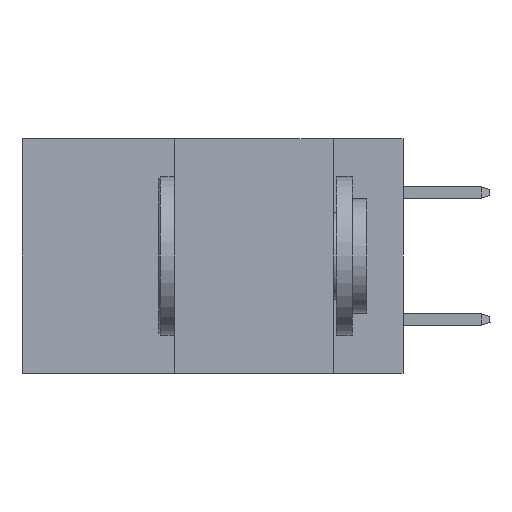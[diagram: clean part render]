
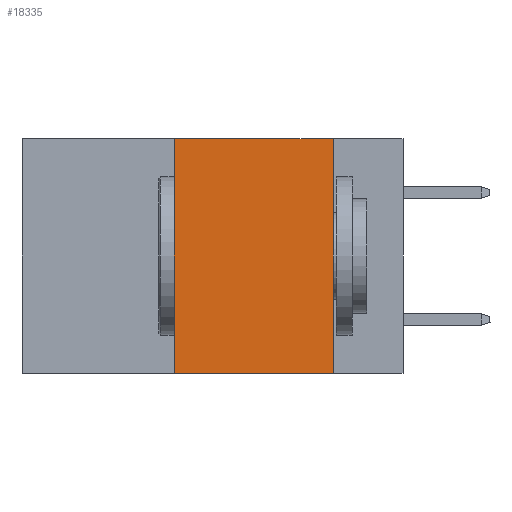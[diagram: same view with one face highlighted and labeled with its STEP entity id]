
A CAD part, left-side view. The second image highlights one B-rep face of the part: STEP entity #18335.
In plain terms, the highlighted planar face has unit normal (-1, 0, 0).
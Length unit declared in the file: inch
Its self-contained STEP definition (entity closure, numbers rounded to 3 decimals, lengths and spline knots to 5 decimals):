
#796 = DIRECTION ( 'NONE',  ( 0., 0., -1. ) ) ;
#1395 = CARTESIAN_POINT ( 'NONE',  ( 0., 0.6, 0. ) ) ;
#2120 = VECTOR ( 'NONE', #17626, 39.37008 ) ;
#2152 = VECTOR ( 'NONE', #2884, 39.37008 ) ;
#2581 = LINE ( 'NONE', #8487, #5072 ) ;
#2884 = DIRECTION ( 'NONE',  ( 0., -1., 0. ) ) ;
#3640 = ORIENTED_EDGE ( 'NONE', *, *, #4110, .F. ) ;
#4110 = EDGE_CURVE ( 'NONE', #10875, #23118, #14291, .T. ) ;
#5072 = VECTOR ( 'NONE', #796, 39.37008 ) ;
#5365 = LINE ( 'NONE', #23094, #23365 ) ;
#5505 = DIRECTION ( 'NONE',  ( 0., -1., 0. ) ) ;
#5621 = DIRECTION ( 'NONE',  ( 0., 0., -1. ) ) ;
#6150 = CARTESIAN_POINT ( 'NONE',  ( 0., 0.36, 0. ) ) ;
#6700 = ORIENTED_EDGE ( 'NONE', *, *, #7539, .F. ) ;
#7539 = EDGE_CURVE ( 'NONE', #16270, #20175, #2581, .T. ) ;
#8487 = CARTESIAN_POINT ( 'NONE',  ( 0., 0.11, 0. ) ) ;
#8534 = CARTESIAN_POINT ( 'NONE',  ( 0., 0.6, -0.37 ) ) ;
#10875 = VERTEX_POINT ( 'NONE', #24563 ) ;
#13480 = EDGE_CURVE ( 'NONE', #10875, #20175, #16751, .T. ) ;
#14291 = LINE ( 'NONE', #20184, #2120 ) ;
#15353 = ORIENTED_EDGE ( 'NONE', *, *, #24662, .F. ) ;
#15500 = PLANE ( 'NONE',  #19904 ) ;
#16270 = VERTEX_POINT ( 'NONE', #23993 ) ;
#16751 = LINE ( 'NONE', #8534, #2152 ) ;
#17626 = DIRECTION ( 'NONE',  ( 0., 0., 1. ) ) ;
#18335 = ADVANCED_FACE ( 'NONE', ( #21014 ), #15500, .F. ) ;
#18361 = EDGE_LOOP ( 'NONE', ( #6700, #15353, #3640, #23550 ) ) ;
#19904 = AXIS2_PLACEMENT_3D ( 'NONE', #1395, #24897, #5621 ) ;
#20175 = VERTEX_POINT ( 'NONE', #21249 ) ;
#20184 = CARTESIAN_POINT ( 'NONE',  ( 0., 0.36, 0. ) ) ;
#21014 = FACE_OUTER_BOUND ( 'NONE', #18361, .T. ) ;
#21249 = CARTESIAN_POINT ( 'NONE',  ( 0., 0.11, -0.37 ) ) ;
#23094 = CARTESIAN_POINT ( 'NONE',  ( 0., 0.6, 0. ) ) ;
#23118 = VERTEX_POINT ( 'NONE', #6150 ) ;
#23365 = VECTOR ( 'NONE', #5505, 39.37008 ) ;
#23550 = ORIENTED_EDGE ( 'NONE', *, *, #13480, .T. ) ;
#23993 = CARTESIAN_POINT ( 'NONE',  ( 0., 0.11, 0. ) ) ;
#24563 = CARTESIAN_POINT ( 'NONE',  ( 0., 0.36, -0.37 ) ) ;
#24662 = EDGE_CURVE ( 'NONE', #23118, #16270, #5365, .T. ) ;
#24897 = DIRECTION ( 'NONE',  ( 1., 0., 0. ) ) ;
